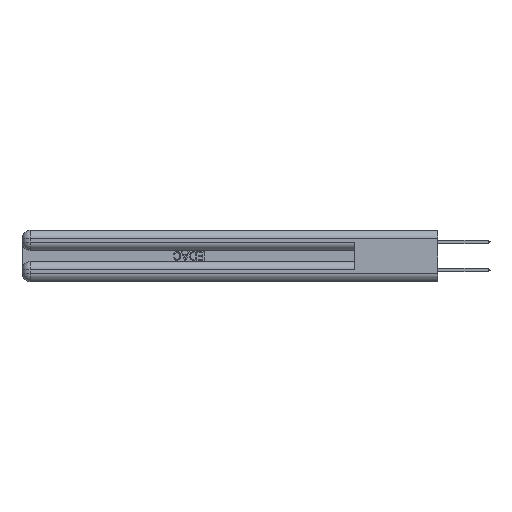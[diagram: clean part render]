
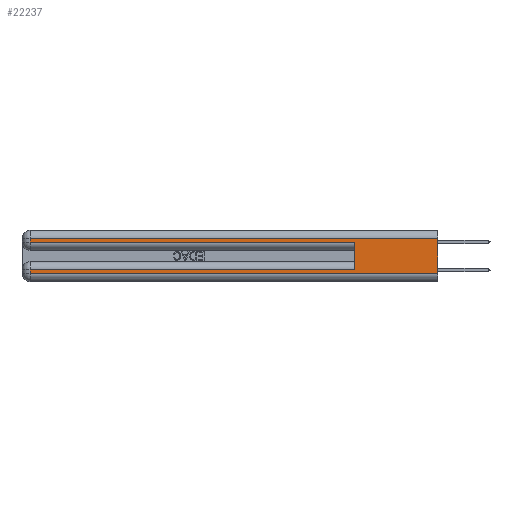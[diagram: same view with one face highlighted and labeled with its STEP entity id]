
A CAD part, left-side view. The second image highlights one B-rep face of the part: STEP entity #22237.
In plain terms, the highlighted planar face has unit normal (-1, 0, 0).
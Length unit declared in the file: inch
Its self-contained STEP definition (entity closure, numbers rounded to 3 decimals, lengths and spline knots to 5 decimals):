
#912 = DIRECTION ( 'NONE',  ( 0., 1., 0. ) ) ;
#1210 = VERTEX_POINT ( 'NONE', #20821 ) ;
#2905 = CARTESIAN_POINT ( 'NONE',  ( 0., 2.94, 0.37 ) ) ;
#3886 = CARTESIAN_POINT ( 'NONE',  ( 0., 2.94, 0.06 ) ) ;
#4258 = CARTESIAN_POINT ( 'NONE',  ( 0., 0., 0.37 ) ) ;
#4535 = VECTOR ( 'NONE', #24083, 39.37008 ) ;
#6963 = EDGE_CURVE ( 'NONE', #20493, #22355, #7544, .T. ) ;
#7057 = VECTOR ( 'NONE', #912, 39.37008 ) ;
#7450 = PLANE ( 'NONE',  #17261 ) ;
#7544 = LINE ( 'NONE', #15494, #38607 ) ;
#7686 = EDGE_CURVE ( 'NONE', #32721, #29498, #29554, .T. ) ;
#8329 = ORIENTED_EDGE ( 'NONE', *, *, #31499, .F. ) ;
#8362 = EDGE_LOOP ( 'NONE', ( #36406, #38403, #13831, #39397, #8329, #11329, #36927, #29415 ) ) ;
#8714 = CARTESIAN_POINT ( 'NONE',  ( 0., 0.6, 0.285 ) ) ;
#9011 = CARTESIAN_POINT ( 'NONE',  ( 0., 2.94, 0.31 ) ) ;
#9295 = CARTESIAN_POINT ( 'NONE',  ( 0., 0., 0.37 ) ) ;
#9921 = LINE ( 'NONE', #37921, #26946 ) ;
#10150 = VERTEX_POINT ( 'NONE', #10578 ) ;
#10578 = CARTESIAN_POINT ( 'NONE',  ( 0., 0.6, 0.085 ) ) ;
#10685 = DIRECTION ( 'NONE',  ( 0., 0., -1. ) ) ;
#10977 = EDGE_CURVE ( 'NONE', #1210, #20493, #38595, .T. ) ;
#11329 = ORIENTED_EDGE ( 'NONE', *, *, #12387, .T. ) ;
#11575 = VERTEX_POINT ( 'NONE', #8714 ) ;
#11857 = FACE_OUTER_BOUND ( 'NONE', #8362, .T. ) ;
#12387 = EDGE_CURVE ( 'NONE', #10150, #1210, #9921, .T. ) ;
#12500 = DIRECTION ( 'NONE',  ( 0., 0., -1. ) ) ;
#12714 = CARTESIAN_POINT ( 'NONE',  ( 0., 0.6, 0.145 ) ) ;
#13831 = ORIENTED_EDGE ( 'NONE', *, *, #7686, .T. ) ;
#14494 = CARTESIAN_POINT ( 'NONE',  ( 0., 0., 0.285 ) ) ;
#15494 = CARTESIAN_POINT ( 'NONE',  ( 0., 0., 0.06 ) ) ;
#16966 = CARTESIAN_POINT ( 'NONE',  ( 0., 0., 0.31 ) ) ;
#17261 = AXIS2_PLACEMENT_3D ( 'NONE', #4258, #29890, #10685 ) ;
#18689 = DIRECTION ( 'NONE',  ( 0., 1., 0. ) ) ;
#18696 = DIRECTION ( 'NONE',  ( 0., -1., 0. ) ) ;
#18823 = LINE ( 'NONE', #9295, #35938 ) ;
#19971 = VECTOR ( 'NONE', #28506, 39.37008 ) ;
#20493 = VERTEX_POINT ( 'NONE', #3886 ) ;
#20821 = CARTESIAN_POINT ( 'NONE',  ( 0., 2.94, 0.085 ) ) ;
#21597 = VECTOR ( 'NONE', #22353, 39.37008 ) ;
#22237 = ADVANCED_FACE ( 'NONE', ( #11857 ), #7450, .F. ) ;
#22353 = DIRECTION ( 'NONE',  ( 0., 0., 1. ) ) ;
#22355 = VERTEX_POINT ( 'NONE', #33645 ) ;
#23627 = LINE ( 'NONE', #12714, #21597 ) ;
#24083 = DIRECTION ( 'NONE',  ( 0., 0., -1. ) ) ;
#24176 = DIRECTION ( 'NONE',  ( 0., -1., 0. ) ) ;
#24616 = EDGE_CURVE ( 'NONE', #37132, #32721, #33603, .T. ) ;
#26946 = VECTOR ( 'NONE', #18689, 39.37008 ) ;
#28506 = DIRECTION ( 'NONE',  ( 0., 0., -1. ) ) ;
#28953 = VECTOR ( 'NONE', #24176, 39.37008 ) ;
#29415 = ORIENTED_EDGE ( 'NONE', *, *, #6963, .T. ) ;
#29498 = VERTEX_POINT ( 'NONE', #40164 ) ;
#29554 = LINE ( 'NONE', #2905, #19971 ) ;
#29890 = DIRECTION ( 'NONE',  ( 1., 0., 0. ) ) ;
#31285 = CARTESIAN_POINT ( 'NONE',  ( 0., 0., 0.31 ) ) ;
#31499 = EDGE_CURVE ( 'NONE', #10150, #11575, #23627, .T. ) ;
#32721 = VERTEX_POINT ( 'NONE', #9011 ) ;
#33603 = LINE ( 'NONE', #16966, #7057 ) ;
#33645 = CARTESIAN_POINT ( 'NONE',  ( 0., 0., 0.06 ) ) ;
#34580 = EDGE_CURVE ( 'NONE', #37132, #22355, #18823, .T. ) ;
#35938 = VECTOR ( 'NONE', #12500, 39.37008 ) ;
#36406 = ORIENTED_EDGE ( 'NONE', *, *, #34580, .F. ) ;
#36414 = EDGE_CURVE ( 'NONE', #29498, #11575, #38463, .T. ) ;
#36848 = CARTESIAN_POINT ( 'NONE',  ( 0., 2.94, 0.37 ) ) ;
#36927 = ORIENTED_EDGE ( 'NONE', *, *, #10977, .T. ) ;
#37132 = VERTEX_POINT ( 'NONE', #31285 ) ;
#37921 = CARTESIAN_POINT ( 'NONE',  ( 0., 0., 0.085 ) ) ;
#38403 = ORIENTED_EDGE ( 'NONE', *, *, #24616, .T. ) ;
#38463 = LINE ( 'NONE', #14494, #28953 ) ;
#38595 = LINE ( 'NONE', #36848, #4535 ) ;
#38607 = VECTOR ( 'NONE', #18696, 39.37008 ) ;
#39397 = ORIENTED_EDGE ( 'NONE', *, *, #36414, .T. ) ;
#40164 = CARTESIAN_POINT ( 'NONE',  ( 0., 2.94, 0.285 ) ) ;
